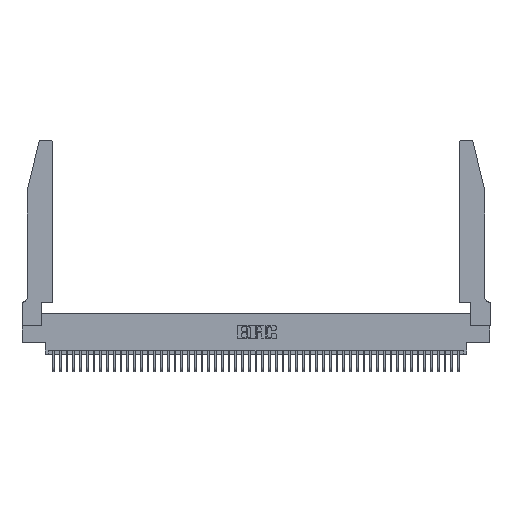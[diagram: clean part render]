
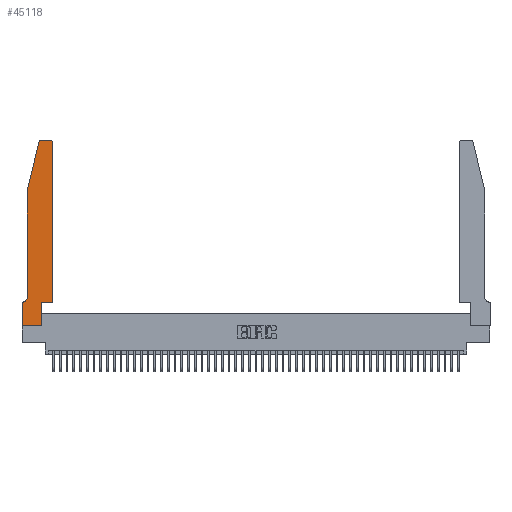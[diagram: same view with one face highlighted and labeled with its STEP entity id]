
A CAD part, top view. The second image highlights one B-rep face of the part: STEP entity #45118.
In plain terms, the highlighted planar face has unit normal (0, 0, 1).
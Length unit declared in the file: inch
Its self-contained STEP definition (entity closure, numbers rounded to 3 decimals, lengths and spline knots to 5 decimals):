
#1161 = ORIENTED_EDGE ( 'NONE', *, *, #29385, .T. ) ;
#1511 = AXIS2_PLACEMENT_3D ( 'NONE', #25221, #40169, #17910 ) ;
#1542 = DIRECTION ( 'NONE',  ( 1., 0., 0. ) ) ;
#1596 = CARTESIAN_POINT ( 'NONE',  ( 0.0755, 0.35, 0.37 ) ) ;
#1759 = DIRECTION ( 'NONE',  ( -1., 0., 0. ) ) ;
#2027 = CARTESIAN_POINT ( 'NONE',  ( 0.2865, 0.35, 0.37 ) ) ;
#3012 = VECTOR ( 'NONE', #1542, 39.37008 ) ;
#3558 = DIRECTION ( 'NONE',  ( 0., 0., 1. ) ) ;
#4627 = EDGE_CURVE ( 'NONE', #23829, #7508, #38275, .T. ) ;
#4747 = DIRECTION ( 'NONE',  ( 1., 0., 0. ) ) ;
#6609 = PLANE ( 'NONE',  #1511 ) ;
#6933 = LINE ( 'NONE', #8145, #15747 ) ;
#7508 = VERTEX_POINT ( 'NONE', #46141 ) ;
#8087 = VERTEX_POINT ( 'NONE', #2027 ) ;
#8145 = CARTESIAN_POINT ( 'NONE',  ( 0., 0., 0.37 ) ) ;
#8642 = VECTOR ( 'NONE', #29260, 39.37008 ) ;
#8750 = CIRCLE ( 'NONE', #30349, 0.07 ) ;
#10082 = CARTESIAN_POINT ( 'NONE',  ( 0.4505, 2.72, 0.37 ) ) ;
#10576 = CARTESIAN_POINT ( 'NONE',  ( 0.2865, 0., 0.37 ) ) ;
#10597 = VERTEX_POINT ( 'NONE', #32521 ) ;
#11481 = VECTOR ( 'NONE', #40749, 39.37008 ) ;
#11946 = DIRECTION ( 'NONE',  ( 0., -1., 0. ) ) ;
#13012 = LINE ( 'NONE', #46200, #3012 ) ;
#13907 = CARTESIAN_POINT ( 'NONE',  ( 0.0055, 0.35, 0.37 ) ) ;
#14587 = CARTESIAN_POINT ( 'NONE',  ( 0.0755, 2., 0.37 ) ) ;
#15711 = CARTESIAN_POINT ( 'NONE',  ( 0.0755, 2., 0.37 ) ) ;
#15747 = VECTOR ( 'NONE', #11946, 39.37008 ) ;
#15883 = ORIENTED_EDGE ( 'NONE', *, *, #34023, .T. ) ;
#16048 = DIRECTION ( 'NONE',  ( 0., 0., -1. ) ) ;
#16340 = ORIENTED_EDGE ( 'NONE', *, *, #21282, .T. ) ;
#16836 = CARTESIAN_POINT ( 'NONE',  ( 0.0755, 2., 0.37 ) ) ;
#17910 = DIRECTION ( 'NONE',  ( 1., 0., 0. ) ) ;
#18157 = VERTEX_POINT ( 'NONE', #35121 ) ;
#18617 = LINE ( 'NONE', #47603, #8642 ) ;
#19103 = EDGE_CURVE ( 'NONE', #26581, #46203, #39928, .T. ) ;
#20190 = CARTESIAN_POINT ( 'NONE',  ( 0.4505, 0.35, 0.37 ) ) ;
#20292 = ORIENTED_EDGE ( 'NONE', *, *, #43497, .T. ) ;
#20967 = CARTESIAN_POINT ( 'NONE',  ( 0.4205, 2.72, 0.37 ) ) ;
#21282 = EDGE_CURVE ( 'NONE', #8087, #24300, #13012, .T. ) ;
#21342 = FACE_OUTER_BOUND ( 'NONE', #33464, .T. ) ;
#21425 = LINE ( 'NONE', #14587, #11481 ) ;
#21689 = LINE ( 'NONE', #36778, #37939 ) ;
#22095 = CIRCLE ( 'NONE', #27780, 0.03 ) ;
#22147 = ORIENTED_EDGE ( 'NONE', *, *, #42131, .T. ) ;
#23030 = DIRECTION ( 'NONE',  ( -0.239, -0.971, 0. ) ) ;
#23415 = CARTESIAN_POINT ( 'NONE',  ( 0., 0., 0.37 ) ) ;
#23829 = VERTEX_POINT ( 'NONE', #13907 ) ;
#24300 = VERTEX_POINT ( 'NONE', #20190 ) ;
#24694 = DIRECTION ( 'NONE',  ( 1., 0., 0. ) ) ;
#25221 = CARTESIAN_POINT ( 'NONE',  ( 0., 0.35, 0.37 ) ) ;
#25237 = ORIENTED_EDGE ( 'NONE', *, *, #19103, .T. ) ;
#25564 = LINE ( 'NONE', #23415, #36612 ) ;
#25584 = ORIENTED_EDGE ( 'NONE', *, *, #4627, .T. ) ;
#25961 = CARTESIAN_POINT ( 'NONE',  ( 0.284, 2.72, 0.37 ) ) ;
#26581 = VERTEX_POINT ( 'NONE', #43500 ) ;
#26594 = DIRECTION ( 'NONE',  ( 0., 1., 0. ) ) ;
#26859 = VECTOR ( 'NONE', #26594, 39.37008 ) ;
#27068 = ORIENTED_EDGE ( 'NONE', *, *, #43963, .T. ) ;
#27780 = AXIS2_PLACEMENT_3D ( 'NONE', #25961, #3558, #29707 ) ;
#27808 = EDGE_CURVE ( 'NONE', #40850, #8087, #18617, .T. ) ;
#29027 = EDGE_CURVE ( 'NONE', #29786, #46161, #35359, .T. ) ;
#29260 = DIRECTION ( 'NONE',  ( 0., 1., 0. ) ) ;
#29385 = EDGE_CURVE ( 'NONE', #7508, #34222, #6933, .T. ) ;
#29707 = DIRECTION ( 'NONE',  ( 1., 0., 0. ) ) ;
#29786 = VERTEX_POINT ( 'NONE', #10082 ) ;
#30208 = ORIENTED_EDGE ( 'NONE', *, *, #40366, .T. ) ;
#30341 = ORIENTED_EDGE ( 'NONE', *, *, #27808, .T. ) ;
#30349 = AXIS2_PLACEMENT_3D ( 'NONE', #38297, #16048, #42056 ) ;
#31916 = ORIENTED_EDGE ( 'NONE', *, *, #29027, .T. ) ;
#32521 = CARTESIAN_POINT ( 'NONE',  ( 0.0755, 0.42, 0.37 ) ) ;
#33464 = EDGE_LOOP ( 'NONE', ( #45944, #27068, #25237, #30208, #15883, #25584, #1161, #20292, #30341, #16340, #22147, #31916 ) ) ;
#33560 = VECTOR ( 'NONE', #23030, 39.37008 ) ;
#33828 = EDGE_CURVE ( 'NONE', #46161, #18157, #21689, .T. ) ;
#34023 = EDGE_CURVE ( 'NONE', #10597, #23829, #8750, .T. ) ;
#34222 = VERTEX_POINT ( 'NONE', #47044 ) ;
#35035 = CARTESIAN_POINT ( 'NONE',  ( 0.4205, 2.75, 0.37 ) ) ;
#35121 = CARTESIAN_POINT ( 'NONE',  ( 0.284, 2.75, 0.37 ) ) ;
#35359 = CIRCLE ( 'NONE', #40798, 0.03 ) ;
#36612 = VECTOR ( 'NONE', #4747, 39.37008 ) ;
#36778 = CARTESIAN_POINT ( 'NONE',  ( 0.2605, 2.75, 0.37 ) ) ;
#37939 = VECTOR ( 'NONE', #40515, 39.37008 ) ;
#38275 = LINE ( 'NONE', #1596, #39449 ) ;
#38297 = CARTESIAN_POINT ( 'NONE',  ( 0.0055, 0.42, 0.37 ) ) ;
#39449 = VECTOR ( 'NONE', #1759, 39.37008 ) ;
#39928 = LINE ( 'NONE', #15711, #33560 ) ;
#40169 = DIRECTION ( 'NONE',  ( 0., 0., 1. ) ) ;
#40366 = EDGE_CURVE ( 'NONE', #46203, #10597, #21425, .T. ) ;
#40515 = DIRECTION ( 'NONE',  ( -1., 0., 0. ) ) ;
#40749 = DIRECTION ( 'NONE',  ( 0., -1., 0. ) ) ;
#40798 = AXIS2_PLACEMENT_3D ( 'NONE', #20967, #46935, #24694 ) ;
#40850 = VERTEX_POINT ( 'NONE', #10576 ) ;
#41389 = CARTESIAN_POINT ( 'NONE',  ( 0.4505, 0.35, 0.37 ) ) ;
#42056 = DIRECTION ( 'NONE',  ( -1., 0., 0. ) ) ;
#42131 = EDGE_CURVE ( 'NONE', #24300, #29786, #46631, .T. ) ;
#43497 = EDGE_CURVE ( 'NONE', #34222, #40850, #25564, .T. ) ;
#43500 = CARTESIAN_POINT ( 'NONE',  ( 0.25487, 2.72718, 0.37 ) ) ;
#43963 = EDGE_CURVE ( 'NONE', #18157, #26581, #22095, .T. ) ;
#45118 = ADVANCED_FACE ( 'NONE', ( #21342 ), #6609, .T. ) ;
#45944 = ORIENTED_EDGE ( 'NONE', *, *, #33828, .T. ) ;
#46141 = CARTESIAN_POINT ( 'NONE',  ( 0., 0.35, 0.37 ) ) ;
#46161 = VERTEX_POINT ( 'NONE', #35035 ) ;
#46200 = CARTESIAN_POINT ( 'NONE',  ( 0.4505, 0.35, 0.37 ) ) ;
#46203 = VERTEX_POINT ( 'NONE', #16836 ) ;
#46631 = LINE ( 'NONE', #41389, #26859 ) ;
#46935 = DIRECTION ( 'NONE',  ( 0., 0., 1. ) ) ;
#47044 = CARTESIAN_POINT ( 'NONE',  ( 0., 0., 0.37 ) ) ;
#47603 = CARTESIAN_POINT ( 'NONE',  ( 0.2865, 0.35, 0.37 ) ) ;
